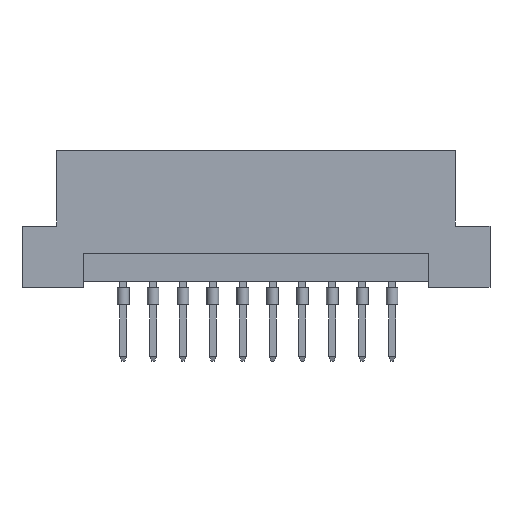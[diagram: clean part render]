
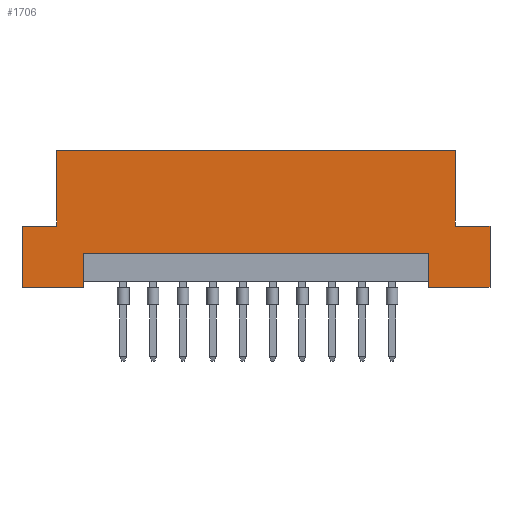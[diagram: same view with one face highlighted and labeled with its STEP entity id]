
A CAD part, front view. The second image highlights one B-rep face of the part: STEP entity #1706.
In plain terms, the highlighted planar face has unit normal (0, -1, 0).
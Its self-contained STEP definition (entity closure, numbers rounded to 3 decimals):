
#26 = CARTESIAN_POINT ( 'NONE',  ( 16.94, 0., 5.2 ) ) ;
#111 = EDGE_CURVE ( 'NONE', #2037, #2703, #5635, .T. ) ;
#172 = ORIENTED_EDGE ( 'NONE', *, *, #4965, .F. ) ;
#371 = VERTEX_POINT ( 'NONE', #1990 ) ;
#391 = DIRECTION ( 'NONE',  ( 0., 0., -1. ) ) ;
#526 = CARTESIAN_POINT ( 'NONE',  ( -19.9, 0., 0. ) ) ;
#585 = LINE ( 'NONE', #26, #1987 ) ;
#826 = VECTOR ( 'NONE', #1524, 1000. ) ;
#970 = EDGE_LOOP ( 'NONE', ( #2252, #4189, #5274, #3894, #2267, #2045, #1574, #3087, #1565, #3460, #172, #5236 ) ) ;
#1042 = CARTESIAN_POINT ( 'NONE',  ( 16.94, 0., 11.6 ) ) ;
#1051 = VECTOR ( 'NONE', #1893, 1000. ) ;
#1076 = CARTESIAN_POINT ( 'NONE',  ( -19.9, 0., 5.2 ) ) ;
#1183 = CARTESIAN_POINT ( 'NONE',  ( -19.9, 0., 5.2 ) ) ;
#1229 = DIRECTION ( 'NONE',  ( -1., 0., 0. ) ) ;
#1250 = DIRECTION ( 'NONE',  ( 0., 0., 1. ) ) ;
#1268 = VERTEX_POINT ( 'NONE', #2190 ) ;
#1372 = CARTESIAN_POINT ( 'NONE',  ( -14.69, 0., 0.5 ) ) ;
#1446 = LINE ( 'NONE', #3043, #5147 ) ;
#1524 = DIRECTION ( 'NONE',  ( 1., 0., 0. ) ) ;
#1558 = VERTEX_POINT ( 'NONE', #5075 ) ;
#1565 = ORIENTED_EDGE ( 'NONE', *, *, #6485, .F. ) ;
#1574 = ORIENTED_EDGE ( 'NONE', *, *, #3366, .F. ) ;
#1706 = ADVANCED_FACE ( 'NONE', ( #3824 ), #4764, .F. ) ;
#1731 = LINE ( 'NONE', #1076, #3094 ) ;
#1854 = CARTESIAN_POINT ( 'NONE',  ( 19.9, 0., 5.2 ) ) ;
#1889 = EDGE_CURVE ( 'NONE', #1268, #371, #4489, .T. ) ;
#1893 = DIRECTION ( 'NONE',  ( 0., 0., -1. ) ) ;
#1987 = VECTOR ( 'NONE', #3291, 1000. ) ;
#1990 = CARTESIAN_POINT ( 'NONE',  ( 14.69, 0., 0. ) ) ;
#2037 = VERTEX_POINT ( 'NONE', #5158 ) ;
#2045 = ORIENTED_EDGE ( 'NONE', *, *, #6372, .T. ) ;
#2127 = VECTOR ( 'NONE', #4861, 1000. ) ;
#2181 = VERTEX_POINT ( 'NONE', #2206 ) ;
#2190 = CARTESIAN_POINT ( 'NONE',  ( 14.69, 0., 2.9 ) ) ;
#2206 = CARTESIAN_POINT ( 'NONE',  ( 19.9, 0., 0. ) ) ;
#2218 = VECTOR ( 'NONE', #1250, 1000. ) ;
#2252 = ORIENTED_EDGE ( 'NONE', *, *, #6029, .F. ) ;
#2267 = ORIENTED_EDGE ( 'NONE', *, *, #4575, .F. ) ;
#2512 = VECTOR ( 'NONE', #391, 1000. ) ;
#2648 = DIRECTION ( 'NONE',  ( 0., 1., 0. ) ) ;
#2691 = LINE ( 'NONE', #526, #5471 ) ;
#2700 = CARTESIAN_POINT ( 'NONE',  ( 19.9, 0., 5.2 ) ) ;
#2703 = VERTEX_POINT ( 'NONE', #5946 ) ;
#2828 = CARTESIAN_POINT ( 'NONE',  ( -16.94, 0., 5.2 ) ) ;
#2870 = LINE ( 'NONE', #5995, #5568 ) ;
#3005 = DIRECTION ( 'NONE',  ( 1., 0., 0. ) ) ;
#3043 = CARTESIAN_POINT ( 'NONE',  ( -19.9, 0., 0. ) ) ;
#3087 = ORIENTED_EDGE ( 'NONE', *, *, #111, .F. ) ;
#3094 = VECTOR ( 'NONE', #3198, 1000. ) ;
#3198 = DIRECTION ( 'NONE',  ( 1., 0., 0. ) ) ;
#3291 = DIRECTION ( 'NONE',  ( 0., 0., 1. ) ) ;
#3366 = EDGE_CURVE ( 'NONE', #2703, #4792, #4472, .T. ) ;
#3383 = CARTESIAN_POINT ( 'NONE',  ( 14.69, 0., 0.5 ) ) ;
#3460 = ORIENTED_EDGE ( 'NONE', *, *, #4163, .F. ) ;
#3568 = CARTESIAN_POINT ( 'NONE',  ( 19.9, 0., 0. ) ) ;
#3648 = EDGE_CURVE ( 'NONE', #3791, #2181, #6748, .T. ) ;
#3791 = VERTEX_POINT ( 'NONE', #2700 ) ;
#3814 = CARTESIAN_POINT ( 'NONE',  ( 14.69, 0., 2.9 ) ) ;
#3824 = FACE_OUTER_BOUND ( 'NONE', #970, .T. ) ;
#3894 = ORIENTED_EDGE ( 'NONE', *, *, #3648, .F. ) ;
#3906 = LINE ( 'NONE', #3814, #4120 ) ;
#3967 = VERTEX_POINT ( 'NONE', #1183 ) ;
#4014 = VECTOR ( 'NONE', #3005, 1000. ) ;
#4120 = VECTOR ( 'NONE', #6041, 1000. ) ;
#4163 = EDGE_CURVE ( 'NONE', #5095, #3967, #2691, .T. ) ;
#4189 = ORIENTED_EDGE ( 'NONE', *, *, #1889, .T. ) ;
#4214 = CARTESIAN_POINT ( 'NONE',  ( -14.69, 0., 0. ) ) ;
#4229 = VERTEX_POINT ( 'NONE', #4214 ) ;
#4472 = LINE ( 'NONE', #6376, #826 ) ;
#4489 = LINE ( 'NONE', #3383, #1051 ) ;
#4526 = DIRECTION ( 'NONE',  ( -1., 0., 0. ) ) ;
#4575 = EDGE_CURVE ( 'NONE', #1558, #3791, #5124, .T. ) ;
#4601 = EDGE_CURVE ( 'NONE', #2181, #371, #1446, .T. ) ;
#4681 = EDGE_CURVE ( 'NONE', #6542, #4229, #6160, .T. ) ;
#4764 = PLANE ( 'NONE',  #5313 ) ;
#4792 = VERTEX_POINT ( 'NONE', #1042 ) ;
#4861 = DIRECTION ( 'NONE',  ( 0., 0., -1. ) ) ;
#4965 = EDGE_CURVE ( 'NONE', #4229, #5095, #2870, .T. ) ;
#5075 = CARTESIAN_POINT ( 'NONE',  ( 16.94, 0., 5.2 ) ) ;
#5095 = VERTEX_POINT ( 'NONE', #5723 ) ;
#5124 = LINE ( 'NONE', #1854, #4014 ) ;
#5147 = VECTOR ( 'NONE', #4526, 1000. ) ;
#5158 = CARTESIAN_POINT ( 'NONE',  ( -16.94, 0., 5.2 ) ) ;
#5236 = ORIENTED_EDGE ( 'NONE', *, *, #4681, .F. ) ;
#5274 = ORIENTED_EDGE ( 'NONE', *, *, #4601, .F. ) ;
#5313 = AXIS2_PLACEMENT_3D ( 'NONE', #6281, #2648, #5802 ) ;
#5471 = VECTOR ( 'NONE', #6775, 1000. ) ;
#5568 = VECTOR ( 'NONE', #1229, 1000. ) ;
#5582 = CARTESIAN_POINT ( 'NONE',  ( -14.69, 0., 2.9 ) ) ;
#5635 = LINE ( 'NONE', #2828, #2218 ) ;
#5723 = CARTESIAN_POINT ( 'NONE',  ( -19.9, 0., 0. ) ) ;
#5802 = DIRECTION ( 'NONE',  ( 0., 0., 1. ) ) ;
#5946 = CARTESIAN_POINT ( 'NONE',  ( -16.94, 0., 11.6 ) ) ;
#5995 = CARTESIAN_POINT ( 'NONE',  ( -19.9, 0., 0. ) ) ;
#6029 = EDGE_CURVE ( 'NONE', #1268, #6542, #3906, .T. ) ;
#6041 = DIRECTION ( 'NONE',  ( -1., 0., 0. ) ) ;
#6160 = LINE ( 'NONE', #1372, #2127 ) ;
#6281 = CARTESIAN_POINT ( 'NONE',  ( -19.9, 0., 11.6 ) ) ;
#6372 = EDGE_CURVE ( 'NONE', #1558, #4792, #585, .T. ) ;
#6376 = CARTESIAN_POINT ( 'NONE',  ( -19.9, 0., 11.6 ) ) ;
#6485 = EDGE_CURVE ( 'NONE', #3967, #2037, #1731, .T. ) ;
#6542 = VERTEX_POINT ( 'NONE', #5582 ) ;
#6748 = LINE ( 'NONE', #3568, #2512 ) ;
#6775 = DIRECTION ( 'NONE',  ( 0., 0., 1. ) ) ;
